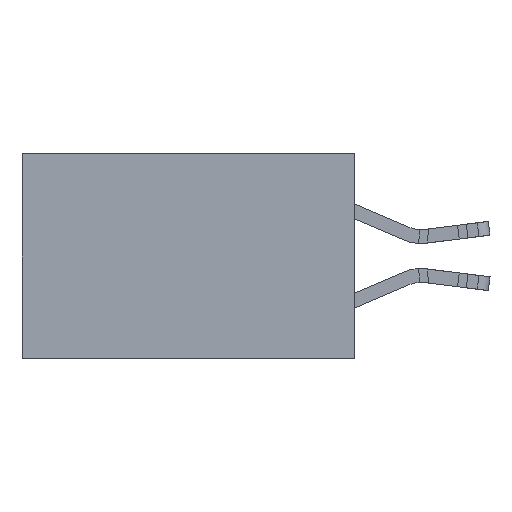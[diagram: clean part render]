
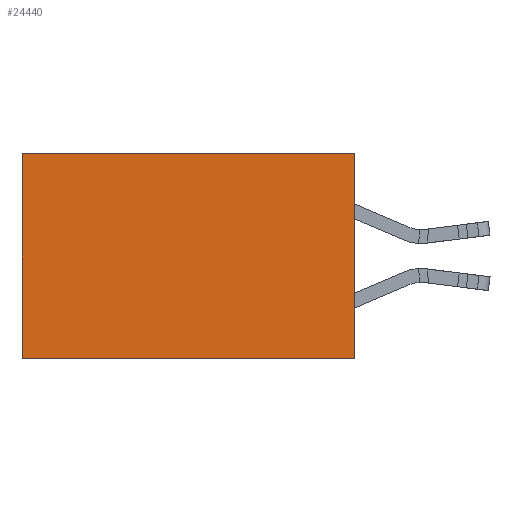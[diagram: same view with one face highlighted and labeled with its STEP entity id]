
A CAD part, left-side view. The second image highlights one B-rep face of the part: STEP entity #24440.
In plain terms, the highlighted planar face has unit normal (-1, 0, 0).
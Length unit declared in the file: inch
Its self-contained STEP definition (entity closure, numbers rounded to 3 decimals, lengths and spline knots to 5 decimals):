
#911 = ORIENTED_EDGE ( 'NONE', *, *, #24444, .T. ) ;
#1285 = DIRECTION ( 'NONE',  ( 0., 0., -1. ) ) ;
#1307 = CARTESIAN_POINT ( 'NONE',  ( 0.2615, 0., -0.37 ) ) ;
#1554 = CARTESIAN_POINT ( 'NONE',  ( 0.2615, 0.6, 0. ) ) ;
#1592 = CARTESIAN_POINT ( 'NONE',  ( 0.2615, 0., 0. ) ) ;
#1671 = CARTESIAN_POINT ( 'NONE',  ( 0.2615, 0., -0.37 ) ) ;
#1745 = DIRECTION ( 'NONE',  ( 1., 0., 0. ) ) ;
#2144 = EDGE_LOOP ( 'NONE', ( #911, #20459, #6053, #18039 ) ) ;
#3281 = EDGE_CURVE ( 'NONE', #5141, #10887, #9419, .T. ) ;
#4894 = FACE_OUTER_BOUND ( 'NONE', #2144, .T. ) ;
#5137 = EDGE_CURVE ( 'NONE', #18829, #5141, #18477, .T. ) ;
#5141 = VERTEX_POINT ( 'NONE', #1671 ) ;
#6053 = ORIENTED_EDGE ( 'NONE', *, *, #5137, .F. ) ;
#7480 = DIRECTION ( 'NONE',  ( 0., 1., 0. ) ) ;
#7642 = DIRECTION ( 'NONE',  ( 0., 0., -1. ) ) ;
#9419 = LINE ( 'NONE', #10095, #19137 ) ;
#9663 = VECTOR ( 'NONE', #7480, 39.37008 ) ;
#10014 = DIRECTION ( 'NONE',  ( 0., 1., 0. ) ) ;
#10060 = VECTOR ( 'NONE', #7642, 39.37008 ) ;
#10095 = CARTESIAN_POINT ( 'NONE',  ( 0.2615, 0., -0.37 ) ) ;
#10887 = VERTEX_POINT ( 'NONE', #11758 ) ;
#11758 = CARTESIAN_POINT ( 'NONE',  ( 0.2615, 0.6, -0.37 ) ) ;
#12710 = VECTOR ( 'NONE', #1285, 39.37008 ) ;
#13407 = EDGE_CURVE ( 'NONE', #18829, #13741, #14883, .T. ) ;
#13431 = CARTESIAN_POINT ( 'NONE',  ( 0.2615, 0., -0.37 ) ) ;
#13543 = CARTESIAN_POINT ( 'NONE',  ( 0.2615, 0., 0. ) ) ;
#13741 = VERTEX_POINT ( 'NONE', #1554 ) ;
#14883 = LINE ( 'NONE', #1592, #9663 ) ;
#15416 = DIRECTION ( 'NONE',  ( 0., 0., -1. ) ) ;
#16600 = AXIS2_PLACEMENT_3D ( 'NONE', #13431, #1745, #15416 ) ;
#18039 = ORIENTED_EDGE ( 'NONE', *, *, #13407, .T. ) ;
#18477 = LINE ( 'NONE', #1307, #12710 ) ;
#18829 = VERTEX_POINT ( 'NONE', #13543 ) ;
#19137 = VECTOR ( 'NONE', #10014, 39.37008 ) ;
#19175 = PLANE ( 'NONE',  #16600 ) ;
#19257 = CARTESIAN_POINT ( 'NONE',  ( 0.2615, 0.6, -0.37 ) ) ;
#20459 = ORIENTED_EDGE ( 'NONE', *, *, #3281, .F. ) ;
#24440 = ADVANCED_FACE ( 'NONE', ( #4894 ), #19175, .F. ) ;
#24444 = EDGE_CURVE ( 'NONE', #13741, #10887, #24793, .T. ) ;
#24793 = LINE ( 'NONE', #19257, #10060 ) ;
